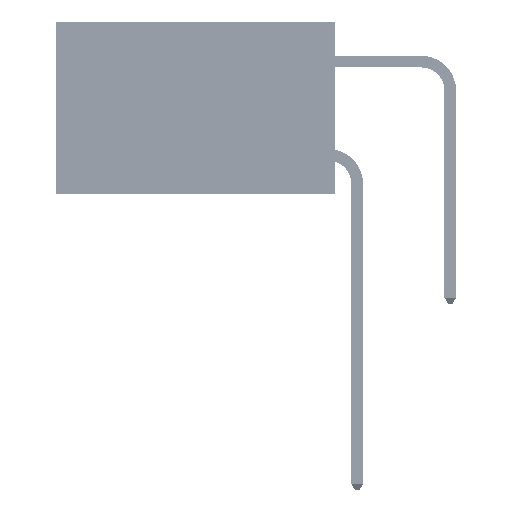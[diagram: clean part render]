
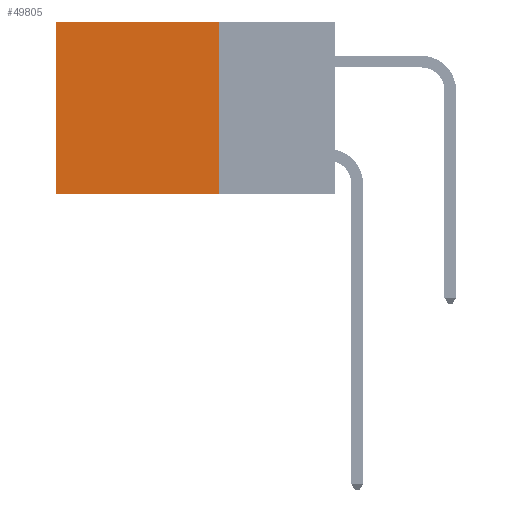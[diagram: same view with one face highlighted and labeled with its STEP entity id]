
A CAD part, left-side view. The second image highlights one B-rep face of the part: STEP entity #49805.
In plain terms, the highlighted planar face has unit normal (-1, 0, 0).
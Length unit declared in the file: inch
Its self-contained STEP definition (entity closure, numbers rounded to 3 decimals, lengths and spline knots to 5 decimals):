
#2301 = VECTOR ( 'NONE', #50019, 39.37008 ) ;
#2480 = DIRECTION ( 'NONE',  ( 0., 0., -1. ) ) ;
#3301 = CARTESIAN_POINT ( 'NONE',  ( 0.2875, 0.25, 0. ) ) ;
#3422 = VECTOR ( 'NONE', #15537, 39.37008 ) ;
#3965 = LINE ( 'NONE', #8728, #15684 ) ;
#4650 = AXIS2_PLACEMENT_3D ( 'NONE', #3301, #41261, #24819 ) ;
#4904 = ORIENTED_EDGE ( 'NONE', *, *, #9701, .F. ) ;
#6576 = LINE ( 'NONE', #23294, #26110 ) ;
#7535 = VERTEX_POINT ( 'NONE', #34490 ) ;
#8093 = EDGE_CURVE ( 'NONE', #49529, #24316, #13434, .T. ) ;
#8728 = CARTESIAN_POINT ( 'NONE',  ( 0.2875, 0.25, 0. ) ) ;
#9701 = EDGE_CURVE ( 'NONE', #12236, #24316, #27570, .T. ) ;
#12236 = VERTEX_POINT ( 'NONE', #15268 ) ;
#12267 = PLANE ( 'NONE',  #4650 ) ;
#13434 = LINE ( 'NONE', #42165, #2301 ) ;
#15268 = CARTESIAN_POINT ( 'NONE',  ( 0.2875, 0.25, -0.37 ) ) ;
#15537 = DIRECTION ( 'NONE',  ( 0., 1., 0. ) ) ;
#15684 = VECTOR ( 'NONE', #25491, 39.37008 ) ;
#22479 = EDGE_CURVE ( 'NONE', #7535, #12236, #6576, .T. ) ;
#23294 = CARTESIAN_POINT ( 'NONE',  ( 0.2875, 0.25, 0. ) ) ;
#24316 = VERTEX_POINT ( 'NONE', #42884 ) ;
#24819 = DIRECTION ( 'NONE',  ( 0., 0., -1. ) ) ;
#25491 = DIRECTION ( 'NONE',  ( 0., 1., 0. ) ) ;
#26110 = VECTOR ( 'NONE', #2480, 39.37008 ) ;
#27570 = LINE ( 'NONE', #45103, #3422 ) ;
#33045 = ORIENTED_EDGE ( 'NONE', *, *, #22479, .F. ) ;
#34185 = ORIENTED_EDGE ( 'NONE', *, *, #35734, .T. ) ;
#34490 = CARTESIAN_POINT ( 'NONE',  ( 0.2875, 0.25, 0. ) ) ;
#34685 = CARTESIAN_POINT ( 'NONE',  ( 0.2875, 0.6, 0. ) ) ;
#35734 = EDGE_CURVE ( 'NONE', #7535, #49529, #3965, .T. ) ;
#38217 = FACE_OUTER_BOUND ( 'NONE', #40010, .T. ) ;
#40010 = EDGE_LOOP ( 'NONE', ( #52102, #4904, #33045, #34185 ) ) ;
#41261 = DIRECTION ( 'NONE',  ( 1., 0., 0. ) ) ;
#42165 = CARTESIAN_POINT ( 'NONE',  ( 0.2875, 0.6, 0. ) ) ;
#42884 = CARTESIAN_POINT ( 'NONE',  ( 0.2875, 0.6, -0.37 ) ) ;
#45103 = CARTESIAN_POINT ( 'NONE',  ( 0.2875, 0.25, -0.37 ) ) ;
#49529 = VERTEX_POINT ( 'NONE', #34685 ) ;
#49805 = ADVANCED_FACE ( 'NONE', ( #38217 ), #12267, .F. ) ;
#50019 = DIRECTION ( 'NONE',  ( 0., 0., -1. ) ) ;
#52102 = ORIENTED_EDGE ( 'NONE', *, *, #8093, .T. ) ;
